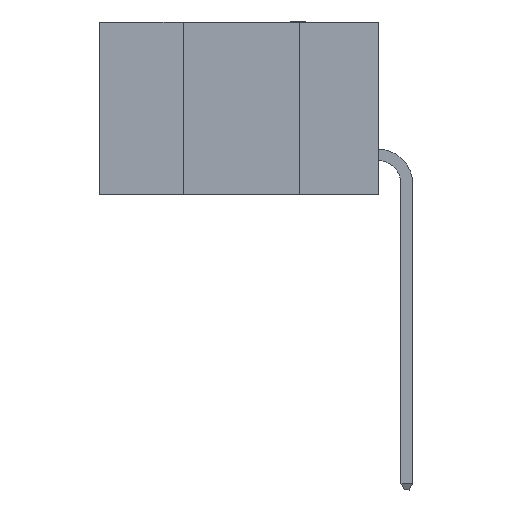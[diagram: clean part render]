
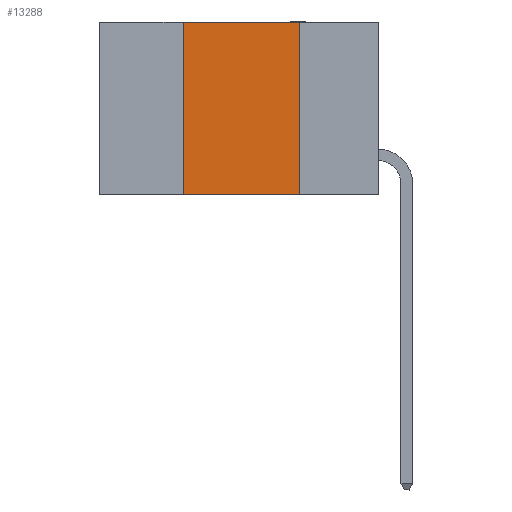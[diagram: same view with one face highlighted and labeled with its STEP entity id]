
A CAD part, left-side view. The second image highlights one B-rep face of the part: STEP entity #13288.
In plain terms, the highlighted planar face has unit normal (-1, 0, 0).
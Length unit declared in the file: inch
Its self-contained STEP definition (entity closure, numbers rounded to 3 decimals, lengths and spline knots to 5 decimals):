
#1546 = DIRECTION ( 'NONE',  ( 0., 0., -1. ) ) ;
#1816 = VECTOR ( 'NONE', #3920, 39.37008 ) ;
#3920 = DIRECTION ( 'NONE',  ( 0., 0., 1. ) ) ;
#5634 = CARTESIAN_POINT ( 'NONE',  ( 0., 0.6, 0. ) ) ;
#6613 = LINE ( 'NONE', #5634, #12691 ) ;
#7765 = VERTEX_POINT ( 'NONE', #26176 ) ;
#7803 = CARTESIAN_POINT ( 'NONE',  ( 0., 0.6, 0. ) ) ;
#8090 = CARTESIAN_POINT ( 'NONE',  ( 0., 0.17, -0.37 ) ) ;
#8114 = CARTESIAN_POINT ( 'NONE',  ( 0., 0.6, -0.37 ) ) ;
#8241 = EDGE_CURVE ( 'NONE', #24566, #10839, #18959, .T. ) ;
#9366 = ORIENTED_EDGE ( 'NONE', *, *, #21492, .F. ) ;
#9705 = DIRECTION ( 'NONE',  ( 0., -1., 0. ) ) ;
#9932 = LINE ( 'NONE', #10945, #25641 ) ;
#10221 = CARTESIAN_POINT ( 'NONE',  ( 0., 0.42, -0.37 ) ) ;
#10839 = VERTEX_POINT ( 'NONE', #8090 ) ;
#10945 = CARTESIAN_POINT ( 'NONE',  ( 0., 0.17, 0. ) ) ;
#11629 = EDGE_CURVE ( 'NONE', #7765, #12777, #6613, .T. ) ;
#12049 = CARTESIAN_POINT ( 'NONE',  ( 0., 0.42, 0. ) ) ;
#12691 = VECTOR ( 'NONE', #9705, 39.37008 ) ;
#12777 = VERTEX_POINT ( 'NONE', #16953 ) ;
#13288 = ADVANCED_FACE ( 'NONE', ( #19941 ), #22009, .F. ) ;
#15339 = AXIS2_PLACEMENT_3D ( 'NONE', #7803, #15805, #1546 ) ;
#15805 = DIRECTION ( 'NONE',  ( 1., 0., 0. ) ) ;
#16953 = CARTESIAN_POINT ( 'NONE',  ( 0., 0.17, 0. ) ) ;
#17331 = DIRECTION ( 'NONE',  ( 0., 0., -1. ) ) ;
#18173 = LINE ( 'NONE', #12049, #1816 ) ;
#18959 = LINE ( 'NONE', #8114, #26304 ) ;
#19941 = FACE_OUTER_BOUND ( 'NONE', #22647, .T. ) ;
#20587 = ORIENTED_EDGE ( 'NONE', *, *, #11629, .F. ) ;
#21492 = EDGE_CURVE ( 'NONE', #24566, #7765, #18173, .T. ) ;
#22009 = PLANE ( 'NONE',  #15339 ) ;
#22192 = ORIENTED_EDGE ( 'NONE', *, *, #8241, .T. ) ;
#22647 = EDGE_LOOP ( 'NONE', ( #25260, #20587, #9366, #22192 ) ) ;
#24438 = DIRECTION ( 'NONE',  ( 0., -1., 0. ) ) ;
#24566 = VERTEX_POINT ( 'NONE', #10221 ) ;
#25229 = EDGE_CURVE ( 'NONE', #12777, #10839, #9932, .T. ) ;
#25260 = ORIENTED_EDGE ( 'NONE', *, *, #25229, .F. ) ;
#25641 = VECTOR ( 'NONE', #17331, 39.37008 ) ;
#26176 = CARTESIAN_POINT ( 'NONE',  ( 0., 0.42, 0. ) ) ;
#26304 = VECTOR ( 'NONE', #24438, 39.37008 ) ;
